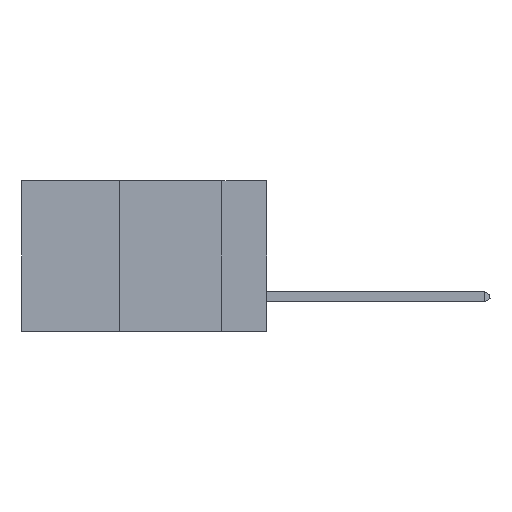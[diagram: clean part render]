
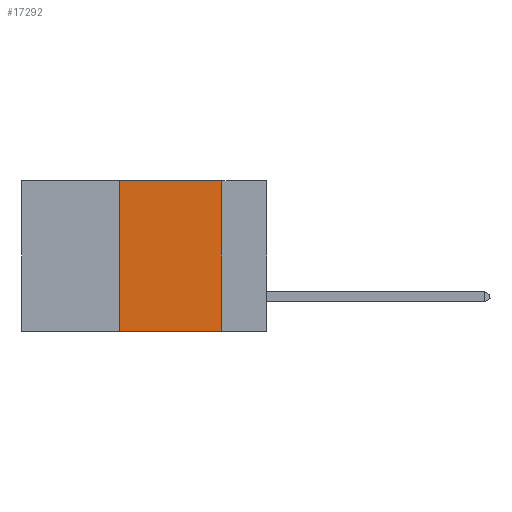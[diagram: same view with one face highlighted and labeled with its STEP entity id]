
A CAD part, left-side view. The second image highlights one B-rep face of the part: STEP entity #17292.
In plain terms, the highlighted planar face has unit normal (-1, 0, 0).
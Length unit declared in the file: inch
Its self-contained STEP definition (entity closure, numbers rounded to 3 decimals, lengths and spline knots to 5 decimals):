
#22 = CARTESIAN_POINT ( 'NONE',  ( 0., 0.6, -0.37 ) ) ;
#375 = EDGE_CURVE ( 'NONE', #6184, #2039, #6518, .T. ) ;
#710 = EDGE_LOOP ( 'NONE', ( #12651, #11886, #8892, #8555 ) ) ;
#1333 = CARTESIAN_POINT ( 'NONE',  ( 0., 0.6, 0. ) ) ;
#2039 = VERTEX_POINT ( 'NONE', #6728 ) ;
#2066 = VERTEX_POINT ( 'NONE', #16189 ) ;
#2287 = LINE ( 'NONE', #6858, #4379 ) ;
#2651 = PLANE ( 'NONE',  #12399 ) ;
#3585 = EDGE_CURVE ( 'NONE', #2039, #10501, #9792, .T. ) ;
#3592 = CARTESIAN_POINT ( 'NONE',  ( 0., 0.6, 0. ) ) ;
#4379 = VECTOR ( 'NONE', #5508, 39.37008 ) ;
#5235 = DIRECTION ( 'NONE',  ( 0., -1., 0. ) ) ;
#5508 = DIRECTION ( 'NONE',  ( 0., 0., -1. ) ) ;
#6184 = VERTEX_POINT ( 'NONE', #16694 ) ;
#6518 = LINE ( 'NONE', #13014, #14978 ) ;
#6728 = CARTESIAN_POINT ( 'NONE',  ( 0., 0.36, 0. ) ) ;
#6858 = CARTESIAN_POINT ( 'NONE',  ( 0., 0.11, 0. ) ) ;
#8037 = CARTESIAN_POINT ( 'NONE',  ( 0., 0.11, 0. ) ) ;
#8259 = VECTOR ( 'NONE', #5235, 39.37008 ) ;
#8555 = ORIENTED_EDGE ( 'NONE', *, *, #13073, .T. ) ;
#8892 = ORIENTED_EDGE ( 'NONE', *, *, #375, .F. ) ;
#9792 = LINE ( 'NONE', #3592, #13607 ) ;
#10154 = LINE ( 'NONE', #22, #8259 ) ;
#10188 = FACE_OUTER_BOUND ( 'NONE', #710, .T. ) ;
#10233 = DIRECTION ( 'NONE',  ( 0., -1., 0. ) ) ;
#10501 = VERTEX_POINT ( 'NONE', #8037 ) ;
#10767 = DIRECTION ( 'NONE',  ( 1., 0., 0. ) ) ;
#11234 = DIRECTION ( 'NONE',  ( 0., 0., -1. ) ) ;
#11707 = DIRECTION ( 'NONE',  ( 0., 0., 1. ) ) ;
#11886 = ORIENTED_EDGE ( 'NONE', *, *, #3585, .F. ) ;
#12399 = AXIS2_PLACEMENT_3D ( 'NONE', #1333, #10767, #11234 ) ;
#12651 = ORIENTED_EDGE ( 'NONE', *, *, #14838, .F. ) ;
#13014 = CARTESIAN_POINT ( 'NONE',  ( 0., 0.36, 0. ) ) ;
#13073 = EDGE_CURVE ( 'NONE', #6184, #2066, #10154, .T. ) ;
#13607 = VECTOR ( 'NONE', #10233, 39.37008 ) ;
#14838 = EDGE_CURVE ( 'NONE', #10501, #2066, #2287, .T. ) ;
#14978 = VECTOR ( 'NONE', #11707, 39.37008 ) ;
#16189 = CARTESIAN_POINT ( 'NONE',  ( 0., 0.11, -0.37 ) ) ;
#16694 = CARTESIAN_POINT ( 'NONE',  ( 0., 0.36, -0.37 ) ) ;
#17292 = ADVANCED_FACE ( 'NONE', ( #10188 ), #2651, .F. ) ;
